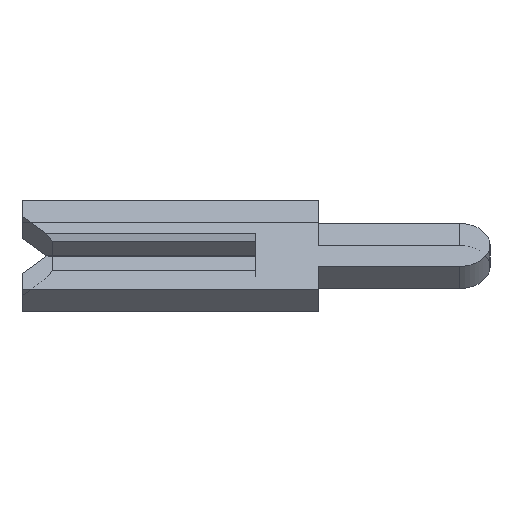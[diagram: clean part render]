
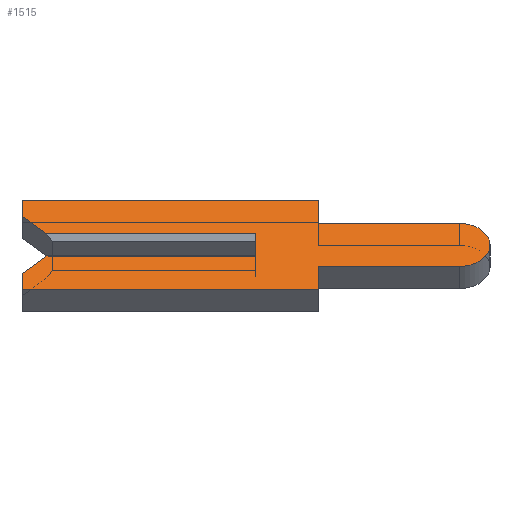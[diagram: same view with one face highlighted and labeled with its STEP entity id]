
A CAD part, left-side view. The second image highlights one B-rep face of the part: STEP entity #1515.
In plain terms, the highlighted face is planar.
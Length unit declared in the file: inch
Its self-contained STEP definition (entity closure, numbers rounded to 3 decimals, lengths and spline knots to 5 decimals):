
#99 = CARTESIAN_POINT ( 'NONE',  ( -0.01, 0.134, -0.01 ) ) ;
#102 = ORIENTED_EDGE ( 'NONE', *, *, #271, .F. ) ;
#122 = CARTESIAN_POINT ( 'NONE',  ( -0.01, -0.04, -0.04 ) ) ;
#137 = CARTESIAN_POINT ( 'NONE',  ( -0.01, -0.1305, 0. ) ) ;
#150 = EDGE_CURVE ( 'NONE', #739, #1753, #2082, .T. ) ;
#198 = CARTESIAN_POINT ( 'NONE',  ( -0.01, 0.15, 0.026 ) ) ;
#210 = EDGE_CURVE ( 'NONE', #2273, #1821, #2776, .T. ) ;
#238 = CARTESIAN_POINT ( 'NONE',  ( -0.01, 0., 0.0065 ) ) ;
#239 = LINE ( 'NONE', #2463, #2467 ) ;
#245 = VECTOR ( 'NONE', #1118, 39.37008 ) ;
#248 = ORIENTED_EDGE ( 'NONE', *, *, #2363, .F. ) ;
#271 = EDGE_CURVE ( 'NONE', #1968, #1547, #1776, .T. ) ;
#289 = ORIENTED_EDGE ( 'NONE', *, *, #1727, .F. ) ;
#301 = CARTESIAN_POINT ( 'NONE',  ( -0.01, -0.1305, 0. ) ) ;
#323 = VECTOR ( 'NONE', #2361, 39.37008 ) ;
#330 = ORIENTED_EDGE ( 'NONE', *, *, #1378, .F. ) ;
#352 = VECTOR ( 'NONE', #1449, 39.37008 ) ;
#414 = EDGE_CURVE ( 'NONE', #1753, #2273, #1433, .T. ) ;
#507 = VECTOR ( 'NONE', #2736, 39.37008 ) ;
#521 = CARTESIAN_POINT ( 'NONE',  ( -0.01, 0.15, 0.04 ) ) ;
#540 = VECTOR ( 'NONE', #1859, 39.37008 ) ;
#552 = AXIS2_PLACEMENT_3D ( 'NONE', #137, #2537, #3002 ) ;
#555 = EDGE_LOOP ( 'NONE', ( #1589, #2564, #696, #2667, #2174, #330, #248, #102, #289, #1438, #735, #2942, #1264, #2247 ) ) ;
#587 = DIRECTION ( 'NONE',  ( 0., -1., 0. ) ) ;
#650 = CARTESIAN_POINT ( 'NONE',  ( -0.01, 0.15, -0.026 ) ) ;
#689 = CIRCLE ( 'NONE', #552, 0.0195 ) ;
#696 = ORIENTED_EDGE ( 'NONE', *, *, #1646, .F. ) ;
#735 = ORIENTED_EDGE ( 'NONE', *, *, #210, .F. ) ;
#739 = VERTEX_POINT ( 'NONE', #1907 ) ;
#742 = LINE ( 'NONE', #238, #1173 ) ;
#748 = DIRECTION ( 'NONE',  ( 0., 1., 0. ) ) ;
#774 = VERTEX_POINT ( 'NONE', #1410 ) ;
#776 = CARTESIAN_POINT ( 'NONE',  ( -0.01, 0.15, -0.04 ) ) ;
#780 = EDGE_CURVE ( 'NONE', #1632, #2129, #742, .T. ) ;
#816 = CARTESIAN_POINT ( 'NONE',  ( -0.01, -0.04, 0.0195 ) ) ;
#859 = LINE ( 'NONE', #2818, #540 ) ;
#904 = CARTESIAN_POINT ( 'NONE',  ( -0.01, -0.04, -0.0195 ) ) ;
#950 = EDGE_CURVE ( 'NONE', #1139, #2169, #239, .T. ) ;
#994 = DIRECTION ( 'NONE',  ( 1., 0., 0. ) ) ;
#1030 = DIRECTION ( 'NONE',  ( 0., 0., 1. ) ) ;
#1045 = CARTESIAN_POINT ( 'NONE',  ( -0.01, 0.15, 0.04 ) ) ;
#1054 = CARTESIAN_POINT ( 'NONE',  ( -0.01, -0.1305, -0.01 ) ) ;
#1084 = LINE ( 'NONE', #2039, #1653 ) ;
#1118 = DIRECTION ( 'NONE',  ( 0., 0., -1. ) ) ;
#1139 = VERTEX_POINT ( 'NONE', #1734 ) ;
#1173 = VECTOR ( 'NONE', #1030, 39.37008 ) ;
#1212 = VECTOR ( 'NONE', #748, 39.37008 ) ;
#1264 = ORIENTED_EDGE ( 'NONE', *, *, #150, .F. ) ;
#1356 = DIRECTION ( 'NONE',  ( 0., 0., -1. ) ) ;
#1378 = EDGE_CURVE ( 'NONE', #1851, #1593, #1499, .T. ) ;
#1410 = CARTESIAN_POINT ( 'NONE',  ( -0.01, -0.1305, 0.0195 ) ) ;
#1433 = LINE ( 'NONE', #521, #352 ) ;
#1438 = ORIENTED_EDGE ( 'NONE', *, *, #1979, .F. ) ;
#1449 = DIRECTION ( 'NONE',  ( 0., -1., 0. ) ) ;
#1499 = LINE ( 'NONE', #776, #1212 ) ;
#1515 = ADVANCED_FACE ( 'NONE', ( #2382 ), #2490, .F. ) ;
#1527 = CARTESIAN_POINT ( 'NONE',  ( -0.01, -0.04, -0.0195 ) ) ;
#1532 = CARTESIAN_POINT ( 'NONE',  ( -0.01, -0.04, 0.04 ) ) ;
#1540 = VECTOR ( 'NONE', #1850, 39.37008 ) ;
#1547 = VERTEX_POINT ( 'NONE', #1527 ) ;
#1589 = ORIENTED_EDGE ( 'NONE', *, *, #2718, .T. ) ;
#1593 = VERTEX_POINT ( 'NONE', #2274 ) ;
#1616 = VECTOR ( 'NONE', #1356, 39.37008 ) ;
#1632 = VERTEX_POINT ( 'NONE', #2528 ) ;
#1646 = EDGE_CURVE ( 'NONE', #2169, #1632, #2621, .T. ) ;
#1653 = VECTOR ( 'NONE', #2009, 39.37008 ) ;
#1727 = EDGE_CURVE ( 'NONE', #774, #1968, #689, .T. ) ;
#1734 = CARTESIAN_POINT ( 'NONE',  ( -0.01, 0.15, -0.026 ) ) ;
#1753 = VERTEX_POINT ( 'NONE', #1045 ) ;
#1758 = DIRECTION ( 'NONE',  ( 0., -0.707, 0.707 ) ) ;
#1761 = CARTESIAN_POINT ( 'NONE',  ( -0.01, -0.1305, -0.0195 ) ) ;
#1776 = LINE ( 'NONE', #904, #323 ) ;
#1821 = VERTEX_POINT ( 'NONE', #816 ) ;
#1850 = DIRECTION ( 'NONE',  ( 0., 0., 1. ) ) ;
#1851 = VERTEX_POINT ( 'NONE', #122 ) ;
#1859 = DIRECTION ( 'NONE',  ( 0., -1., 0. ) ) ;
#1905 = VERTEX_POINT ( 'NONE', #2774 ) ;
#1907 = CARTESIAN_POINT ( 'NONE',  ( -0.01, 0.15, 0.026 ) ) ;
#1916 = AXIS2_PLACEMENT_3D ( 'NONE', #301, #994, #2218 ) ;
#1968 = VERTEX_POINT ( 'NONE', #1761 ) ;
#1979 = EDGE_CURVE ( 'NONE', #1821, #774, #1084, .T. ) ;
#2009 = DIRECTION ( 'NONE',  ( 0., -1., 0. ) ) ;
#2039 = CARTESIAN_POINT ( 'NONE',  ( -0.01, -0.04, 0.0195 ) ) ;
#2041 = VECTOR ( 'NONE', #587, 39.37008 ) ;
#2072 = LINE ( 'NONE', #2583, #1616 ) ;
#2082 = LINE ( 'NONE', #198, #1540 ) ;
#2129 = VERTEX_POINT ( 'NONE', #2250 ) ;
#2169 = VERTEX_POINT ( 'NONE', #99 ) ;
#2174 = ORIENTED_EDGE ( 'NONE', *, *, #2535, .F. ) ;
#2218 = DIRECTION ( 'NONE',  ( 0., 0., -1. ) ) ;
#2247 = ORIENTED_EDGE ( 'NONE', *, *, #2783, .F. ) ;
#2250 = CARTESIAN_POINT ( 'NONE',  ( -0.01, 0., 0.01 ) ) ;
#2273 = VERTEX_POINT ( 'NONE', #1532 ) ;
#2274 = CARTESIAN_POINT ( 'NONE',  ( -0.01, 0.15, -0.04 ) ) ;
#2302 = CARTESIAN_POINT ( 'NONE',  ( -0.01, 0.1305, 0.0065 ) ) ;
#2335 = DIRECTION ( 'NONE',  ( 0., 0., 1. ) ) ;
#2361 = DIRECTION ( 'NONE',  ( 0., 1., 0. ) ) ;
#2363 = EDGE_CURVE ( 'NONE', #1547, #1851, #2072, .T. ) ;
#2382 = FACE_OUTER_BOUND ( 'NONE', #555, .T. ) ;
#2463 = CARTESIAN_POINT ( 'NONE',  ( -0.01, 0.1305, -0.0065 ) ) ;
#2464 = LINE ( 'NONE', #2302, #507 ) ;
#2467 = VECTOR ( 'NONE', #1758, 39.37008 ) ;
#2490 = PLANE ( 'NONE',  #1916 ) ;
#2528 = CARTESIAN_POINT ( 'NONE',  ( -0.01, 0., -0.01 ) ) ;
#2535 = EDGE_CURVE ( 'NONE', #1593, #1139, #2975, .T. ) ;
#2537 = DIRECTION ( 'NONE',  ( 1., 0., 0. ) ) ;
#2564 = ORIENTED_EDGE ( 'NONE', *, *, #780, .F. ) ;
#2583 = CARTESIAN_POINT ( 'NONE',  ( -0.01, -0.04, -0.04 ) ) ;
#2615 = CARTESIAN_POINT ( 'NONE',  ( -0.01, -0.04, 0.04 ) ) ;
#2621 = LINE ( 'NONE', #1054, #2041 ) ;
#2667 = ORIENTED_EDGE ( 'NONE', *, *, #950, .F. ) ;
#2718 = EDGE_CURVE ( 'NONE', #1905, #2129, #859, .T. ) ;
#2736 = DIRECTION ( 'NONE',  ( 0., 0.707, 0.707 ) ) ;
#2772 = VECTOR ( 'NONE', #2335, 39.37008 ) ;
#2774 = CARTESIAN_POINT ( 'NONE',  ( -0.01, 0.134, 0.01 ) ) ;
#2776 = LINE ( 'NONE', #2615, #245 ) ;
#2783 = EDGE_CURVE ( 'NONE', #1905, #739, #2464, .T. ) ;
#2818 = CARTESIAN_POINT ( 'NONE',  ( -0.01, 0.15, 0.01 ) ) ;
#2942 = ORIENTED_EDGE ( 'NONE', *, *, #414, .F. ) ;
#2975 = LINE ( 'NONE', #650, #2772 ) ;
#3002 = DIRECTION ( 'NONE',  ( 0., 0., -1. ) ) ;
